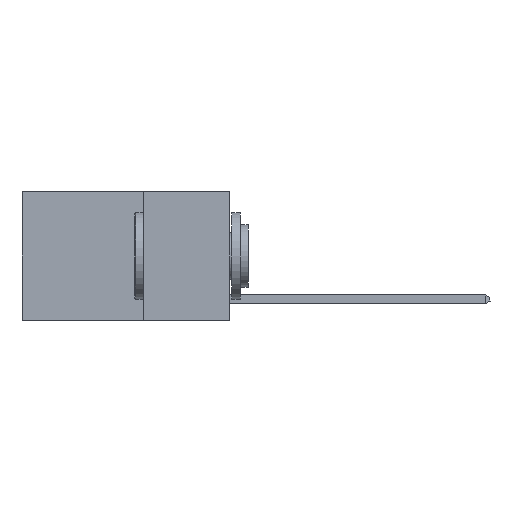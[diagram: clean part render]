
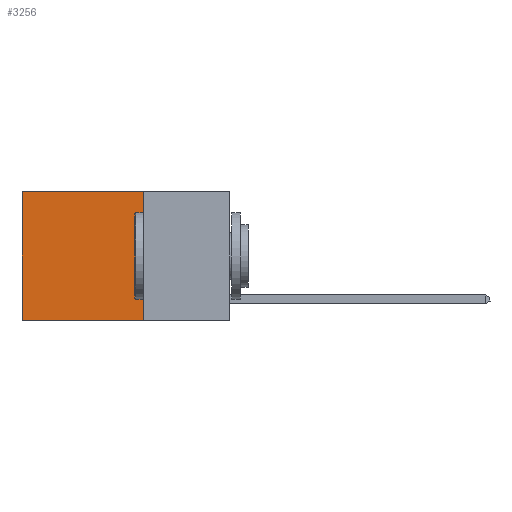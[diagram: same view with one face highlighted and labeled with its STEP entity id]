
A CAD part, left-side view. The second image highlights one B-rep face of the part: STEP entity #3256.
In plain terms, the highlighted planar face has unit normal (-1, 0, 0).
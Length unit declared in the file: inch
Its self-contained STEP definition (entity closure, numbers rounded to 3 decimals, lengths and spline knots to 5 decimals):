
#504 = AXIS2_PLACEMENT_3D ( 'NONE', #4110, #14369, #5572 ) ;
#561 = CARTESIAN_POINT ( 'NONE',  ( 0.2625, 0.25, 0. ) ) ;
#1278 = ORIENTED_EDGE ( 'NONE', *, *, #14659, .F. ) ;
#1338 = VERTEX_POINT ( 'NONE', #8264 ) ;
#1811 = CARTESIAN_POINT ( 'NONE',  ( 0.2625, 0.6, 0. ) ) ;
#1940 = EDGE_LOOP ( 'NONE', ( #6013, #11410, #1278, #18669 ) ) ;
#3256 = ADVANCED_FACE ( 'NONE', ( #11252 ), #18654, .F. ) ;
#4110 = CARTESIAN_POINT ( 'NONE',  ( 0.2625, 0.25, 0. ) ) ;
#5572 = DIRECTION ( 'NONE',  ( 0., 0., -1. ) ) ;
#5754 = CARTESIAN_POINT ( 'NONE',  ( 0.2625, 0.6, -0.37 ) ) ;
#5832 = EDGE_CURVE ( 'NONE', #1338, #10603, #11792, .T. ) ;
#5845 = VECTOR ( 'NONE', #16723, 39.37008 ) ;
#5947 = EDGE_CURVE ( 'NONE', #10239, #14649, #17308, .T. ) ;
#6013 = ORIENTED_EDGE ( 'NONE', *, *, #13076, .T. ) ;
#6848 = CARTESIAN_POINT ( 'NONE',  ( 0.2625, 0.25, 0. ) ) ;
#8002 = CARTESIAN_POINT ( 'NONE',  ( 0.2625, 0.6, 0. ) ) ;
#8133 = DIRECTION ( 'NONE',  ( 0., 1., 0. ) ) ;
#8264 = CARTESIAN_POINT ( 'NONE',  ( 0.2625, 0.25, -0.37 ) ) ;
#8386 = DIRECTION ( 'NONE',  ( 0., 1., 0. ) ) ;
#10239 = VERTEX_POINT ( 'NONE', #561 ) ;
#10603 = VERTEX_POINT ( 'NONE', #5754 ) ;
#11252 = FACE_OUTER_BOUND ( 'NONE', #1940, .T. ) ;
#11410 = ORIENTED_EDGE ( 'NONE', *, *, #5832, .F. ) ;
#11792 = LINE ( 'NONE', #18346, #15266 ) ;
#12111 = DIRECTION ( 'NONE',  ( 0., 0., -1. ) ) ;
#13076 = EDGE_CURVE ( 'NONE', #14649, #10603, #17525, .T. ) ;
#13430 = VECTOR ( 'NONE', #8386, 39.37008 ) ;
#13827 = VECTOR ( 'NONE', #12111, 39.37008 ) ;
#14289 = LINE ( 'NONE', #17932, #13827 ) ;
#14369 = DIRECTION ( 'NONE',  ( 1., 0., 0. ) ) ;
#14649 = VERTEX_POINT ( 'NONE', #1811 ) ;
#14659 = EDGE_CURVE ( 'NONE', #10239, #1338, #14289, .T. ) ;
#15266 = VECTOR ( 'NONE', #8133, 39.37008 ) ;
#16723 = DIRECTION ( 'NONE',  ( 0., 0., -1. ) ) ;
#17308 = LINE ( 'NONE', #6848, #13430 ) ;
#17525 = LINE ( 'NONE', #8002, #5845 ) ;
#17932 = CARTESIAN_POINT ( 'NONE',  ( 0.2625, 0.25, 0. ) ) ;
#18346 = CARTESIAN_POINT ( 'NONE',  ( 0.2625, 0.25, -0.37 ) ) ;
#18654 = PLANE ( 'NONE',  #504 ) ;
#18669 = ORIENTED_EDGE ( 'NONE', *, *, #5947, .T. ) ;
